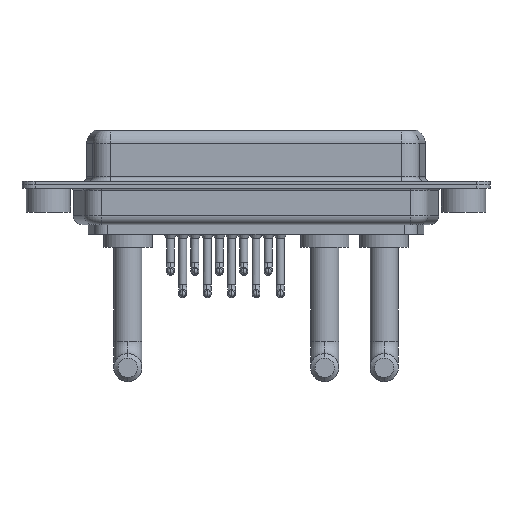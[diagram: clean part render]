
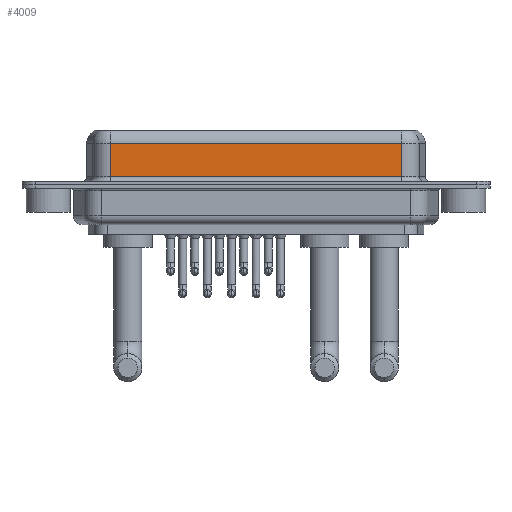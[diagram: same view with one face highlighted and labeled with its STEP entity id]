
A CAD part, front view. The second image highlights one B-rep face of the part: STEP entity #4009.
In plain terms, the highlighted planar face has unit normal (0, -1, 0).
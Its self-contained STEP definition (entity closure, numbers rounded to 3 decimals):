
#444 = DIRECTION ( 'NONE',  ( 0., 0., -1. ) ) ;
#900 = CARTESIAN_POINT ( 'NONE',  ( 40.037, -3.95, 4.65 ) ) ;
#1137 = CARTESIAN_POINT ( 'NONE',  ( 40.037, -3.95, 6.4 ) ) ;
#1273 = CARTESIAN_POINT ( 'NONE',  ( 40.037, -3.95, 0.9 ) ) ;
#1601 = ORIENTED_EDGE ( 'NONE', *, *, #18131, .F. ) ;
#1644 = EDGE_CURVE ( 'NONE', #3694, #7061, #10759, .T. ) ;
#1648 = DIRECTION ( 'NONE',  ( 1., 0., 0. ) ) ;
#1763 = VECTOR ( 'NONE', #6745, 1000. ) ;
#1839 = CARTESIAN_POINT ( 'NONE',  ( 7.013, -3.95, 6.4 ) ) ;
#2585 = PLANE ( 'NONE',  #16389 ) ;
#3110 = VERTEX_POINT ( 'NONE', #900 ) ;
#3694 = VERTEX_POINT ( 'NONE', #9002 ) ;
#4009 = ADVANCED_FACE ( 'NONE', ( #8216 ), #2585, .F. ) ;
#4552 = LINE ( 'NONE', #10472, #17794 ) ;
#6745 = DIRECTION ( 'NONE',  ( -1., 0., 0. ) ) ;
#7061 = VERTEX_POINT ( 'NONE', #17441 ) ;
#8216 = FACE_OUTER_BOUND ( 'NONE', #13421, .T. ) ;
#8498 = VECTOR ( 'NONE', #444, 1000. ) ;
#9002 = CARTESIAN_POINT ( 'NONE',  ( 7.013, -3.95, 4.65 ) ) ;
#9171 = LINE ( 'NONE', #9365, #8498 ) ;
#9365 = CARTESIAN_POINT ( 'NONE',  ( 40.037, -3.95, 6.4 ) ) ;
#10472 = CARTESIAN_POINT ( 'NONE',  ( 40.037, -3.95, 0.9 ) ) ;
#10759 = LINE ( 'NONE', #1839, #13212 ) ;
#11464 = ORIENTED_EDGE ( 'NONE', *, *, #13509, .T. ) ;
#11612 = EDGE_CURVE ( 'NONE', #7061, #16986, #4552, .T. ) ;
#13212 = VECTOR ( 'NONE', #17877, 1000. ) ;
#13421 = EDGE_LOOP ( 'NONE', ( #1601, #11464, #15498, #14131 ) ) ;
#13509 = EDGE_CURVE ( 'NONE', #3110, #3694, #14018, .T. ) ;
#14018 = LINE ( 'NONE', #18432, #1763 ) ;
#14122 = DIRECTION ( 'NONE',  ( 0., 0., 1. ) ) ;
#14131 = ORIENTED_EDGE ( 'NONE', *, *, #11612, .T. ) ;
#15498 = ORIENTED_EDGE ( 'NONE', *, *, #1644, .T. ) ;
#15570 = DIRECTION ( 'NONE',  ( 0., 1., 0. ) ) ;
#16389 = AXIS2_PLACEMENT_3D ( 'NONE', #1137, #15570, #14122 ) ;
#16986 = VERTEX_POINT ( 'NONE', #1273 ) ;
#17441 = CARTESIAN_POINT ( 'NONE',  ( 7.013, -3.95, 0.9 ) ) ;
#17794 = VECTOR ( 'NONE', #1648, 1000. ) ;
#17877 = DIRECTION ( 'NONE',  ( 0., 0., -1. ) ) ;
#18131 = EDGE_CURVE ( 'NONE', #3110, #16986, #9171, .T. ) ;
#18432 = CARTESIAN_POINT ( 'NONE',  ( 40.037, -3.95, 4.65 ) ) ;
